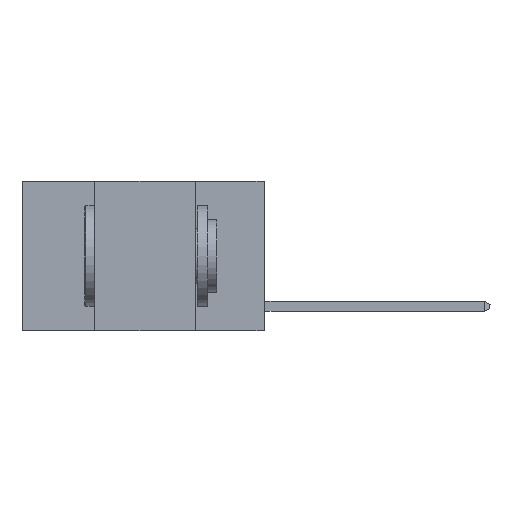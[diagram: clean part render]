
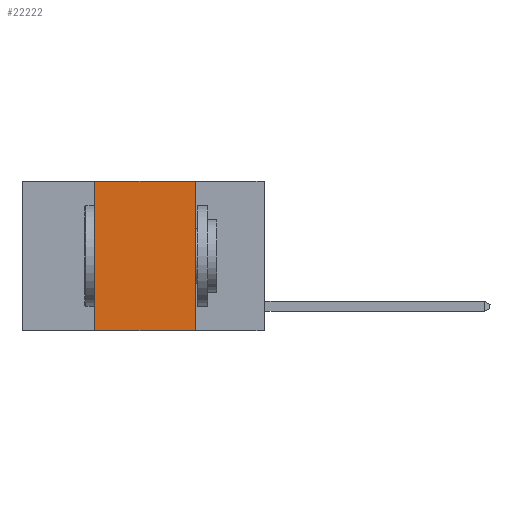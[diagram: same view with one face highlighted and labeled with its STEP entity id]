
A CAD part, left-side view. The second image highlights one B-rep face of the part: STEP entity #22222.
In plain terms, the highlighted planar face has unit normal (-1, 0, 0).
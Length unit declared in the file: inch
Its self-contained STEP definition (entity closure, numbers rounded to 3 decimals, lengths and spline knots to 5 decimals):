
#756 = LINE ( 'NONE', #3528, #26380 ) ;
#777 = ORIENTED_EDGE ( 'NONE', *, *, #25333, .T. ) ;
#1845 = CARTESIAN_POINT ( 'NONE',  ( 0., 0.42, -0.37 ) ) ;
#3528 = CARTESIAN_POINT ( 'NONE',  ( 0., 0.42, 0. ) ) ;
#3617 = CARTESIAN_POINT ( 'NONE',  ( 0., 0.6, -0.37 ) ) ;
#4188 = DIRECTION ( 'NONE',  ( 0., -1., 0. ) ) ;
#5733 = CARTESIAN_POINT ( 'NONE',  ( 0., 0.6, 0. ) ) ;
#6839 = EDGE_CURVE ( 'NONE', #26646, #27149, #756, .T. ) ;
#10031 = DIRECTION ( 'NONE',  ( 0., 0., 1. ) ) ;
#10478 = LINE ( 'NONE', #19577, #12366 ) ;
#10699 = DIRECTION ( 'NONE',  ( 1., 0., 0. ) ) ;
#10808 = VECTOR ( 'NONE', #12645, 39.37008 ) ;
#12134 = CARTESIAN_POINT ( 'NONE',  ( 0., 0.17, 0. ) ) ;
#12366 = VECTOR ( 'NONE', #28594, 39.37008 ) ;
#12645 = DIRECTION ( 'NONE',  ( 0., -1., 0. ) ) ;
#13935 = EDGE_LOOP ( 'NONE', ( #21386, #19978, #21955, #777 ) ) ;
#14232 = VERTEX_POINT ( 'NONE', #12134 ) ;
#14471 = EDGE_CURVE ( 'NONE', #14232, #17255, #10478, .T. ) ;
#17255 = VERTEX_POINT ( 'NONE', #26903 ) ;
#17834 = VECTOR ( 'NONE', #4188, 39.37008 ) ;
#18400 = CARTESIAN_POINT ( 'NONE',  ( 0., 0.6, 0. ) ) ;
#19577 = CARTESIAN_POINT ( 'NONE',  ( 0., 0.17, 0. ) ) ;
#19621 = CARTESIAN_POINT ( 'NONE',  ( 0., 0.42, 0. ) ) ;
#19801 = DIRECTION ( 'NONE',  ( 0., 0., -1. ) ) ;
#19978 = ORIENTED_EDGE ( 'NONE', *, *, #22813, .F. ) ;
#20912 = AXIS2_PLACEMENT_3D ( 'NONE', #5733, #10699, #19801 ) ;
#21386 = ORIENTED_EDGE ( 'NONE', *, *, #14471, .F. ) ;
#21955 = ORIENTED_EDGE ( 'NONE', *, *, #6839, .F. ) ;
#22222 = ADVANCED_FACE ( 'NONE', ( #24377 ), #26627, .F. ) ;
#22813 = EDGE_CURVE ( 'NONE', #27149, #14232, #25359, .T. ) ;
#23947 = LINE ( 'NONE', #3617, #10808 ) ;
#24377 = FACE_OUTER_BOUND ( 'NONE', #13935, .T. ) ;
#25333 = EDGE_CURVE ( 'NONE', #26646, #17255, #23947, .T. ) ;
#25359 = LINE ( 'NONE', #18400, #17834 ) ;
#26380 = VECTOR ( 'NONE', #10031, 39.37008 ) ;
#26627 = PLANE ( 'NONE',  #20912 ) ;
#26646 = VERTEX_POINT ( 'NONE', #1845 ) ;
#26903 = CARTESIAN_POINT ( 'NONE',  ( 0., 0.17, -0.37 ) ) ;
#27149 = VERTEX_POINT ( 'NONE', #19621 ) ;
#28594 = DIRECTION ( 'NONE',  ( 0., 0., -1. ) ) ;
